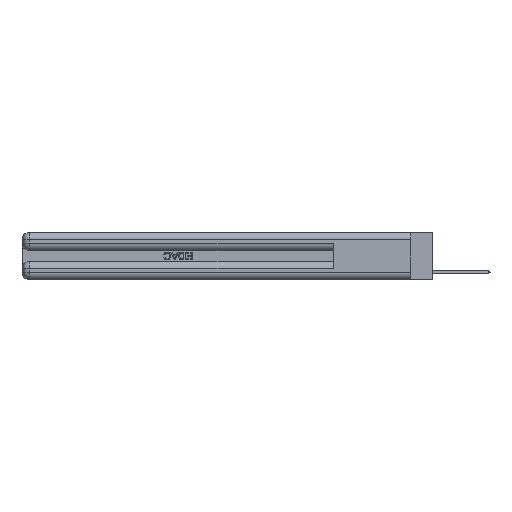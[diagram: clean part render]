
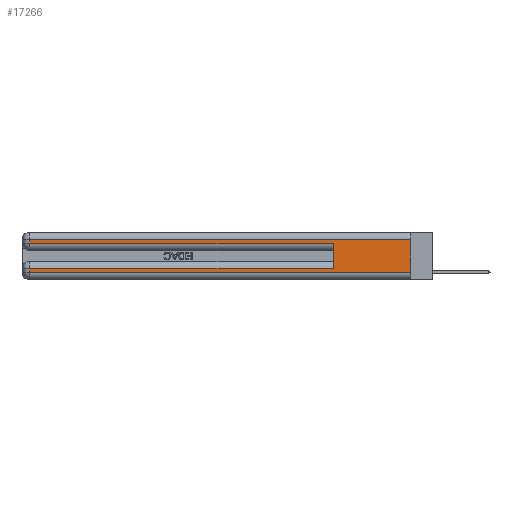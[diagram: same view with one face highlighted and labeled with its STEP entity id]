
A CAD part, left-side view. The second image highlights one B-rep face of the part: STEP entity #17266.
In plain terms, the highlighted planar face has unit normal (-1, 0, 0).
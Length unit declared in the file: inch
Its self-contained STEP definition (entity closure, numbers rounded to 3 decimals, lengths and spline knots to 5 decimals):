
#703 = VECTOR ( 'NONE', #22270, 39.37008 ) ;
#706 = CARTESIAN_POINT ( 'NONE',  ( 0., 0.6, 0.145 ) ) ;
#1420 = VERTEX_POINT ( 'NONE', #24665 ) ;
#1452 = VERTEX_POINT ( 'NONE', #22644 ) ;
#2303 = VECTOR ( 'NONE', #18781, 39.37008 ) ;
#2319 = DIRECTION ( 'NONE',  ( 0., 0., -1. ) ) ;
#2345 = VERTEX_POINT ( 'NONE', #17401 ) ;
#2757 = CARTESIAN_POINT ( 'NONE',  ( 0., 0.6, 0.285 ) ) ;
#2996 = DIRECTION ( 'NONE',  ( 0., -1., 0. ) ) ;
#3138 = CARTESIAN_POINT ( 'NONE',  ( 0., 2.94, 0.285 ) ) ;
#4051 = EDGE_CURVE ( 'NONE', #29926, #1452, #22493, .T. ) ;
#4574 = EDGE_CURVE ( 'NONE', #2345, #6241, #25932, .T. ) ;
#5002 = CARTESIAN_POINT ( 'NONE',  ( 0., 0., 0.285 ) ) ;
#6241 = VERTEX_POINT ( 'NONE', #2757 ) ;
#7277 = CARTESIAN_POINT ( 'NONE',  ( 0., 0., 0.37 ) ) ;
#7447 = DIRECTION ( 'NONE',  ( 1., 0., 0. ) ) ;
#7622 = CARTESIAN_POINT ( 'NONE',  ( 0., 0., 0.37 ) ) ;
#7836 = VERTEX_POINT ( 'NONE', #21030 ) ;
#7997 = VECTOR ( 'NONE', #18801, 39.37008 ) ;
#8130 = ORIENTED_EDGE ( 'NONE', *, *, #4051, .T. ) ;
#8138 = EDGE_CURVE ( 'NONE', #7836, #29159, #29085, .T. ) ;
#8338 = CARTESIAN_POINT ( 'NONE',  ( 0., 0., 0.06 ) ) ;
#8429 = ORIENTED_EDGE ( 'NONE', *, *, #21460, .T. ) ;
#8597 = ORIENTED_EDGE ( 'NONE', *, *, #8138, .T. ) ;
#8658 = CARTESIAN_POINT ( 'NONE',  ( 0., 2.94, 0.37 ) ) ;
#9768 = DIRECTION ( 'NONE',  ( 0., 0., -1. ) ) ;
#10151 = DIRECTION ( 'NONE',  ( 0., 1., 0. ) ) ;
#10473 = CARTESIAN_POINT ( 'NONE',  ( 0., 0., 0.085 ) ) ;
#11753 = ORIENTED_EDGE ( 'NONE', *, *, #4574, .F. ) ;
#12443 = VECTOR ( 'NONE', #28426, 39.37008 ) ;
#13162 = AXIS2_PLACEMENT_3D ( 'NONE', #7277, #7447, #9768 ) ;
#13891 = CARTESIAN_POINT ( 'NONE',  ( 0., 0., 0.06 ) ) ;
#14354 = EDGE_CURVE ( 'NONE', #28622, #6241, #25746, .T. ) ;
#15522 = CARTESIAN_POINT ( 'NONE',  ( 0., 0., 0.31 ) ) ;
#16013 = VECTOR ( 'NONE', #10151, 39.37008 ) ;
#17266 = ADVANCED_FACE ( 'NONE', ( #27372 ), #22703, .F. ) ;
#17301 = EDGE_CURVE ( 'NONE', #29926, #29159, #30359, .T. ) ;
#17401 = CARTESIAN_POINT ( 'NONE',  ( 0., 0.6, 0.085 ) ) ;
#18449 = VECTOR ( 'NONE', #2319, 39.37008 ) ;
#18781 = DIRECTION ( 'NONE',  ( 0., 0., -1. ) ) ;
#18801 = DIRECTION ( 'NONE',  ( 0., -1., 0. ) ) ;
#19801 = ORIENTED_EDGE ( 'NONE', *, *, #17301, .F. ) ;
#20169 = DIRECTION ( 'NONE',  ( 0., 1., 0. ) ) ;
#20778 = ORIENTED_EDGE ( 'NONE', *, *, #24566, .T. ) ;
#21030 = CARTESIAN_POINT ( 'NONE',  ( 0., 2.94, 0.06 ) ) ;
#21460 = EDGE_CURVE ( 'NONE', #2345, #1420, #27592, .T. ) ;
#21480 = VECTOR ( 'NONE', #20169, 39.37008 ) ;
#21726 = ORIENTED_EDGE ( 'NONE', *, *, #14354, .T. ) ;
#22106 = CARTESIAN_POINT ( 'NONE',  ( 0., 2.94, 0.37 ) ) ;
#22270 = DIRECTION ( 'NONE',  ( 0., 0., -1. ) ) ;
#22493 = LINE ( 'NONE', #15522, #21480 ) ;
#22565 = VECTOR ( 'NONE', #2996, 39.37008 ) ;
#22644 = CARTESIAN_POINT ( 'NONE',  ( 0., 2.94, 0.31 ) ) ;
#22703 = PLANE ( 'NONE',  #13162 ) ;
#24566 = EDGE_CURVE ( 'NONE', #1420, #7836, #31404, .T. ) ;
#24665 = CARTESIAN_POINT ( 'NONE',  ( 0., 2.94, 0.085 ) ) ;
#24683 = EDGE_CURVE ( 'NONE', #1452, #28622, #32086, .T. ) ;
#25746 = LINE ( 'NONE', #5002, #22565 ) ;
#25932 = LINE ( 'NONE', #706, #12443 ) ;
#27146 = EDGE_LOOP ( 'NONE', ( #19801, #8130, #28640, #21726, #11753, #8429, #20778, #8597 ) ) ;
#27217 = CARTESIAN_POINT ( 'NONE',  ( 0., 0., 0.31 ) ) ;
#27372 = FACE_OUTER_BOUND ( 'NONE', #27146, .T. ) ;
#27592 = LINE ( 'NONE', #10473, #16013 ) ;
#28426 = DIRECTION ( 'NONE',  ( 0., 0., 1. ) ) ;
#28622 = VERTEX_POINT ( 'NONE', #3138 ) ;
#28640 = ORIENTED_EDGE ( 'NONE', *, *, #24683, .T. ) ;
#29085 = LINE ( 'NONE', #8338, #7997 ) ;
#29159 = VERTEX_POINT ( 'NONE', #13891 ) ;
#29926 = VERTEX_POINT ( 'NONE', #27217 ) ;
#30359 = LINE ( 'NONE', #7622, #18449 ) ;
#31404 = LINE ( 'NONE', #8658, #2303 ) ;
#32086 = LINE ( 'NONE', #22106, #703 ) ;
